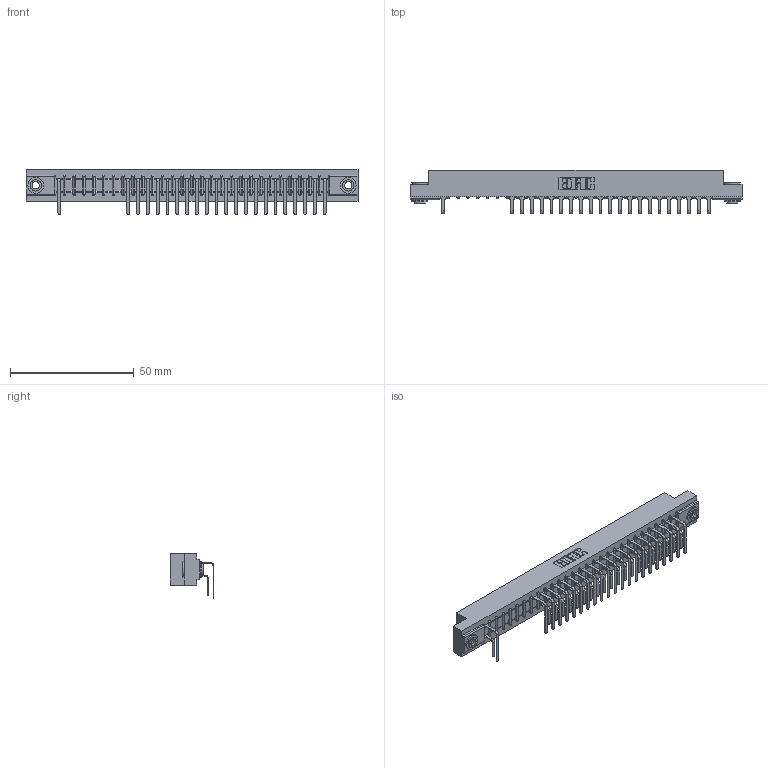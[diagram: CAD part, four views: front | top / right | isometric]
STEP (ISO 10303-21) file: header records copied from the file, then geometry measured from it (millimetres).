
FILE_DESCRIPTION (( 'STEP AP203' ), '1' );
FILE_NAME ('357-028-559-103.STEP', '2018-08-09T05:49:19', ( '' ), ( '' ), 'SwSTEP 2.0', 'SolidWorks 2016', '' );
FILE_SCHEMA (( 'CONFIG_CONTROL_DESIGN' ));
Length unit declared in the file: inch
Products named in the file (5): 307 Part_.156 Dia Mounting Holes; 345-250-002_345-250-002-102; 307-290-001_558 559 - 1 (Single); 357-028-559-103; 307-290-001_559 - 2 (Single)
Assembly tree (46 placements, depth 2):
  357-028-559-103
    307 Part_.156 Dia Mounting Holes
    307-290-001_558 559 - 1 (Single)  x21
    307-290-001_559 - 2 (Single)  x22
    345-250-002_345-250-002-102  x2
Bounding box: 133.96 x 17.69 x 18.07 mm (x, y, z)
Volume: 14171.1 mm3; surface area: 17323.1 mm2
Topology: 46 solids, 46 shells, 2479 faces, 6957 edges, 4498 vertices
Faces by surface type: plane 1591, cylinder 822, sphere 58, cone 8
Entity records: 28722 total; most frequent: CARTESIAN_POINT 4742, ORIENTED_EDGE 4702, DIRECTION 4651, EDGE_CURVE 2351, LINE 1789, VECTOR 1789, VERTEX_POINT 1522, AXIS2_PLACEMENT_3D 1431
